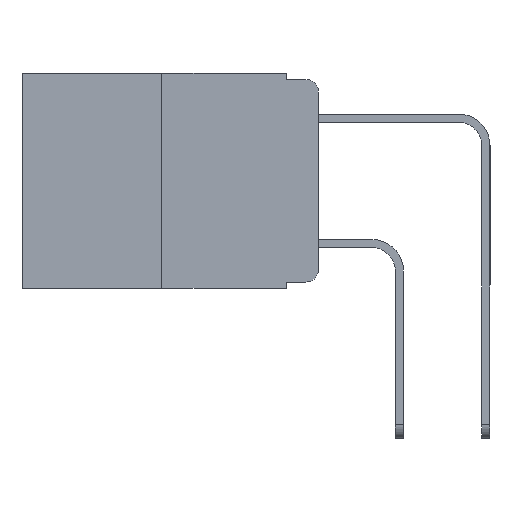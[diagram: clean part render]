
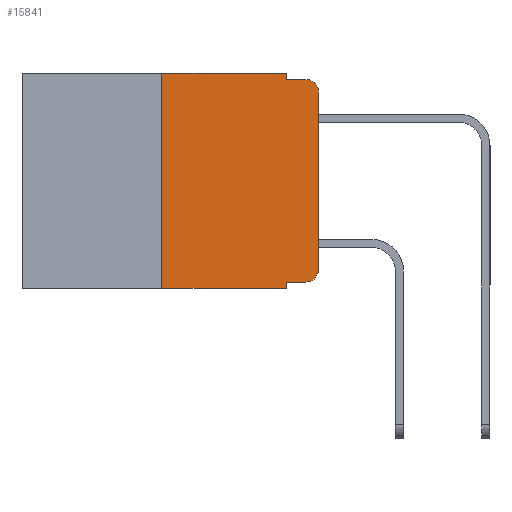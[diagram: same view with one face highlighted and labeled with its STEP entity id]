
A CAD part, left-side view. The second image highlights one B-rep face of the part: STEP entity #15841.
In plain terms, the highlighted planar face has unit normal (-1, 0, 0).
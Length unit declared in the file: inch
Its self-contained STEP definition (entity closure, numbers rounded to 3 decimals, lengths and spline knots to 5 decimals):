
#685 = CARTESIAN_POINT ( 'NONE',  ( 0., 0.02, -0.03 ) ) ;
#807 = VERTEX_POINT ( 'NONE', #6406 ) ;
#973 = LINE ( 'NONE', #6543, #14508 ) ;
#1018 = ORIENTED_EDGE ( 'NONE', *, *, #10884, .F. ) ;
#1177 = CIRCLE ( 'NONE', #7423, 0.02 ) ;
#1252 = ORIENTED_EDGE ( 'NONE', *, *, #8798, .T. ) ;
#1271 = AXIS2_PLACEMENT_3D ( 'NONE', #685, #10083, #2072 ) ;
#1476 = CARTESIAN_POINT ( 'NONE',  ( 0., 0.02, -0.01 ) ) ;
#1583 = FACE_OUTER_BOUND ( 'NONE', #6812, .T. ) ;
#2072 = DIRECTION ( 'NONE',  ( 0., 0., -1. ) ) ;
#2353 = VERTEX_POINT ( 'NONE', #8710 ) ;
#3315 = LINE ( 'NONE', #10928, #12932 ) ;
#3369 = CARTESIAN_POINT ( 'NONE',  ( 0., 0., -0.03 ) ) ;
#3439 = EDGE_CURVE ( 'NONE', #2353, #12681, #4915, .T. ) ;
#3617 = ORIENTED_EDGE ( 'NONE', *, *, #5259, .F. ) ;
#3807 = CARTESIAN_POINT ( 'NONE',  ( 0., 0.051, 0. ) ) ;
#4497 = VERTEX_POINT ( 'NONE', #11946 ) ;
#4871 = CARTESIAN_POINT ( 'NONE',  ( 0., 0.25, -0.343 ) ) ;
#4915 = LINE ( 'NONE', #7389, #15169 ) ;
#5142 = VERTEX_POINT ( 'NONE', #16545 ) ;
#5259 = EDGE_CURVE ( 'NONE', #14020, #4497, #973, .T. ) ;
#5633 = CARTESIAN_POINT ( 'NONE',  ( 0., 0.051, 0. ) ) ;
#5916 = DIRECTION ( 'NONE',  ( 0., 0., 1. ) ) ;
#6160 = EDGE_CURVE ( 'NONE', #5142, #15826, #15257, .T. ) ;
#6210 = DIRECTION ( 'NONE',  ( 1., 0., 0. ) ) ;
#6406 = CARTESIAN_POINT ( 'NONE',  ( 0., 0.051, -0.01 ) ) ;
#6543 = CARTESIAN_POINT ( 'NONE',  ( 0., 0.25, 0. ) ) ;
#6812 = EDGE_LOOP ( 'NONE', ( #15313, #8406, #7997, #1018, #10836, #3617, #16107, #14565, #12220, #1252 ) ) ;
#6968 = VECTOR ( 'NONE', #9785, 39.37008 ) ;
#7389 = CARTESIAN_POINT ( 'NONE',  ( 0., 0., 0. ) ) ;
#7423 = AXIS2_PLACEMENT_3D ( 'NONE', #15296, #7723, #16546 ) ;
#7566 = VERTEX_POINT ( 'NONE', #5633 ) ;
#7723 = DIRECTION ( 'NONE',  ( -1., 0., 0. ) ) ;
#7914 = EDGE_CURVE ( 'NONE', #14020, #15826, #14885, .T. ) ;
#7997 = ORIENTED_EDGE ( 'NONE', *, *, #13812, .F. ) ;
#8406 = ORIENTED_EDGE ( 'NONE', *, *, #9345, .T. ) ;
#8710 = CARTESIAN_POINT ( 'NONE',  ( 0., 0., -0.313 ) ) ;
#8798 = EDGE_CURVE ( 'NONE', #10851, #2353, #1177, .T. ) ;
#9055 = VERTEX_POINT ( 'NONE', #1476 ) ;
#9057 = DIRECTION ( 'NONE',  ( 0., 0., 1. ) ) ;
#9345 = EDGE_CURVE ( 'NONE', #12681, #9055, #10558, .T. ) ;
#9531 = CARTESIAN_POINT ( 'NONE',  ( 0., 0.051, 0. ) ) ;
#9641 = DIRECTION ( 'NONE',  ( 0., -1., 0. ) ) ;
#9785 = DIRECTION ( 'NONE',  ( 0., -1., 0. ) ) ;
#9786 = AXIS2_PLACEMENT_3D ( 'NONE', #13896, #6210, #15136 ) ;
#10083 = DIRECTION ( 'NONE',  ( -1., 0., 0. ) ) ;
#10558 = CIRCLE ( 'NONE', #1271, 0.02 ) ;
#10580 = LINE ( 'NONE', #15429, #13532 ) ;
#10836 = ORIENTED_EDGE ( 'NONE', *, *, #14867, .F. ) ;
#10851 = VERTEX_POINT ( 'NONE', #13232 ) ;
#10884 = EDGE_CURVE ( 'NONE', #7566, #807, #16171, .T. ) ;
#10928 = CARTESIAN_POINT ( 'NONE',  ( 0., 0.051, -0.333 ) ) ;
#11380 = PLANE ( 'NONE',  #9786 ) ;
#11560 = VECTOR ( 'NONE', #14117, 39.37008 ) ;
#11581 = VECTOR ( 'NONE', #14070, 39.37008 ) ;
#11946 = CARTESIAN_POINT ( 'NONE',  ( 0., 0.25, 0. ) ) ;
#12220 = ORIENTED_EDGE ( 'NONE', *, *, #16206, .T. ) ;
#12681 = VERTEX_POINT ( 'NONE', #3369 ) ;
#12877 = VECTOR ( 'NONE', #15831, 39.37008 ) ;
#12932 = VECTOR ( 'NONE', #9641, 39.37008 ) ;
#13232 = CARTESIAN_POINT ( 'NONE',  ( 0., 0.02, -0.333 ) ) ;
#13532 = VECTOR ( 'NONE', #14466, 39.37008 ) ;
#13772 = LINE ( 'NONE', #16023, #6968 ) ;
#13812 = EDGE_CURVE ( 'NONE', #807, #9055, #13772, .T. ) ;
#13896 = CARTESIAN_POINT ( 'NONE',  ( 0., 0.473, 0. ) ) ;
#14020 = VERTEX_POINT ( 'NONE', #4871 ) ;
#14070 = DIRECTION ( 'NONE',  ( 0., -1., 0. ) ) ;
#14117 = DIRECTION ( 'NONE',  ( 0., 0., -1. ) ) ;
#14466 = DIRECTION ( 'NONE',  ( 0., -1., 0. ) ) ;
#14508 = VECTOR ( 'NONE', #5916, 39.37008 ) ;
#14565 = ORIENTED_EDGE ( 'NONE', *, *, #6160, .F. ) ;
#14867 = EDGE_CURVE ( 'NONE', #4497, #7566, #10580, .T. ) ;
#14885 = LINE ( 'NONE', #16504, #11581 ) ;
#15029 = CARTESIAN_POINT ( 'NONE',  ( 0., 0.051, -0.343 ) ) ;
#15136 = DIRECTION ( 'NONE',  ( 0., 0., -1. ) ) ;
#15169 = VECTOR ( 'NONE', #9057, 39.37008 ) ;
#15257 = LINE ( 'NONE', #3807, #11560 ) ;
#15296 = CARTESIAN_POINT ( 'NONE',  ( 0., 0.02, -0.313 ) ) ;
#15313 = ORIENTED_EDGE ( 'NONE', *, *, #3439, .T. ) ;
#15429 = CARTESIAN_POINT ( 'NONE',  ( 0., 0.473, 0. ) ) ;
#15826 = VERTEX_POINT ( 'NONE', #15029 ) ;
#15831 = DIRECTION ( 'NONE',  ( 0., 0., -1. ) ) ;
#15841 = ADVANCED_FACE ( 'NONE', ( #1583 ), #11380, .F. ) ;
#16023 = CARTESIAN_POINT ( 'NONE',  ( 0., 0.051, -0.01 ) ) ;
#16107 = ORIENTED_EDGE ( 'NONE', *, *, #7914, .T. ) ;
#16171 = LINE ( 'NONE', #9531, #12877 ) ;
#16206 = EDGE_CURVE ( 'NONE', #5142, #10851, #3315, .T. ) ;
#16504 = CARTESIAN_POINT ( 'NONE',  ( 0., 0.473, -0.343 ) ) ;
#16545 = CARTESIAN_POINT ( 'NONE',  ( 0., 0.051, -0.333 ) ) ;
#16546 = DIRECTION ( 'NONE',  ( 0., 0., -1. ) ) ;
